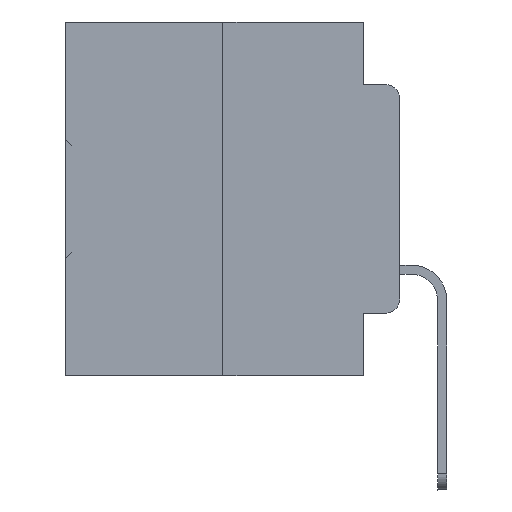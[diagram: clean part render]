
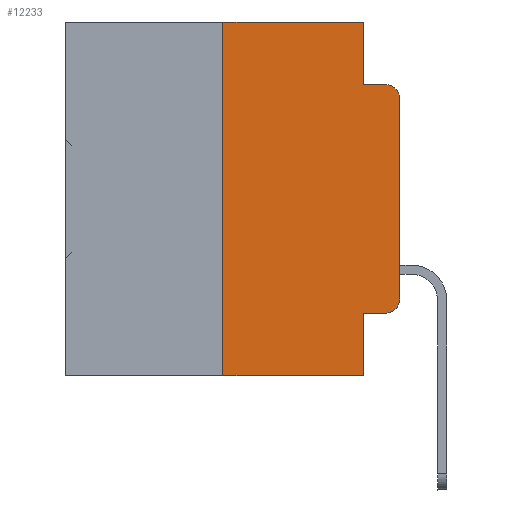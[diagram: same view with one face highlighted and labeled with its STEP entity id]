
A CAD part, left-side view. The second image highlights one B-rep face of the part: STEP entity #12233.
In plain terms, the highlighted planar face has unit normal (-1, 0, 0).
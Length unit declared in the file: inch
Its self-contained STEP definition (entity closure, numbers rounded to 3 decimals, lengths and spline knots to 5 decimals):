
#321 = EDGE_CURVE ( 'NONE', #11624, #19529, #2840, .T. ) ;
#1465 = EDGE_CURVE ( 'NONE', #12386, #24815, #33762, .T. ) ;
#1504 = LINE ( 'NONE', #9749, #30972 ) ;
#1624 = ORIENTED_EDGE ( 'NONE', *, *, #29999, .F. ) ;
#1955 = VERTEX_POINT ( 'NONE', #26578 ) ;
#1976 = ORIENTED_EDGE ( 'NONE', *, *, #26984, .T. ) ;
#2329 = VECTOR ( 'NONE', #22412, 39.37008 ) ;
#2693 = ORIENTED_EDGE ( 'NONE', *, *, #1465, .T. ) ;
#2697 = DIRECTION ( 'NONE',  ( 0., 0., 1. ) ) ;
#2840 = LINE ( 'NONE', #5362, #21229 ) ;
#3437 = EDGE_LOOP ( 'NONE', ( #18092, #22411, #13789, #13077, #34495, #13968, #5350, #1624, #1976, #2693 ) ) ;
#4171 = DIRECTION ( 'NONE',  ( 0., -1., 0. ) ) ;
#4357 = AXIS2_PLACEMENT_3D ( 'NONE', #8572, #22682, #22506 ) ;
#4537 = VECTOR ( 'NONE', #34761, 39.37008 ) ;
#5217 = VECTOR ( 'NONE', #26780, 39.37008 ) ;
#5269 = DIRECTION ( 'NONE',  ( 0., -1., 0. ) ) ;
#5350 = ORIENTED_EDGE ( 'NONE', *, *, #20491, .T. ) ;
#5362 = CARTESIAN_POINT ( 'NONE',  ( 0., 0.473, 0. ) ) ;
#5395 = CARTESIAN_POINT ( 'NONE',  ( 0., 0.25, 0. ) ) ;
#6308 = CARTESIAN_POINT ( 'NONE',  ( 0., 0.051, 0. ) ) ;
#6674 = CARTESIAN_POINT ( 'NONE',  ( 0., 0.051, -0.0885 ) ) ;
#8049 = AXIS2_PLACEMENT_3D ( 'NONE', #9454, #20366, #17683 ) ;
#8396 = DIRECTION ( 'NONE',  ( 0., 0., -1. ) ) ;
#8426 = EDGE_CURVE ( 'NONE', #19529, #9426, #27746, .T. ) ;
#8572 = CARTESIAN_POINT ( 'NONE',  ( 0., 0.02, -0.1085 ) ) ;
#9426 = VERTEX_POINT ( 'NONE', #30774 ) ;
#9454 = CARTESIAN_POINT ( 'NONE',  ( 0., 0.02, -0.3915 ) ) ;
#9749 = CARTESIAN_POINT ( 'NONE',  ( 0., 0.473, -0.5 ) ) ;
#9916 = CARTESIAN_POINT ( 'NONE',  ( 0., 0.051, 0. ) ) ;
#10252 = EDGE_CURVE ( 'NONE', #9426, #20749, #14718, .T. ) ;
#10330 = CARTESIAN_POINT ( 'NONE',  ( 0., 0.051, -0.4115 ) ) ;
#10726 = PLANE ( 'NONE',  #22239 ) ;
#11624 = VERTEX_POINT ( 'NONE', #28161 ) ;
#11834 = VECTOR ( 'NONE', #4171, 39.37008 ) ;
#12233 = ADVANCED_FACE ( 'NONE', ( #16439 ), #10726, .F. ) ;
#12386 = VERTEX_POINT ( 'NONE', #33266 ) ;
#13077 = ORIENTED_EDGE ( 'NONE', *, *, #8426, .F. ) ;
#13789 = ORIENTED_EDGE ( 'NONE', *, *, #10252, .F. ) ;
#13914 = VERTEX_POINT ( 'NONE', #22358 ) ;
#13968 = ORIENTED_EDGE ( 'NONE', *, *, #21806, .F. ) ;
#14221 = VECTOR ( 'NONE', #2697, 39.37008 ) ;
#14718 = LINE ( 'NONE', #6674, #11834 ) ;
#15417 = VERTEX_POINT ( 'NONE', #22706 ) ;
#16270 = DIRECTION ( 'NONE',  ( 0., -1., 0. ) ) ;
#16439 = FACE_OUTER_BOUND ( 'NONE', #3437, .T. ) ;
#17683 = DIRECTION ( 'NONE',  ( 0., 0., -1. ) ) ;
#18092 = ORIENTED_EDGE ( 'NONE', *, *, #19408, .T. ) ;
#18486 = LINE ( 'NONE', #9916, #4537 ) ;
#19408 = EDGE_CURVE ( 'NONE', #24815, #30811, #19719, .T. ) ;
#19529 = VERTEX_POINT ( 'NONE', #6308 ) ;
#19719 = LINE ( 'NONE', #20094, #2329 ) ;
#20094 = CARTESIAN_POINT ( 'NONE',  ( 0., 0., 0. ) ) ;
#20366 = DIRECTION ( 'NONE',  ( -1., 0., 0. ) ) ;
#20491 = EDGE_CURVE ( 'NONE', #13914, #15417, #1504, .T. ) ;
#20749 = VERTEX_POINT ( 'NONE', #30478 ) ;
#21229 = VECTOR ( 'NONE', #16270, 39.37008 ) ;
#21687 = CARTESIAN_POINT ( 'NONE',  ( 0., 0., -0.3915 ) ) ;
#21806 = EDGE_CURVE ( 'NONE', #13914, #11624, #27218, .T. ) ;
#22239 = AXIS2_PLACEMENT_3D ( 'NONE', #30047, #27356, #8396 ) ;
#22358 = CARTESIAN_POINT ( 'NONE',  ( 0., 0.25, -0.5 ) ) ;
#22411 = ORIENTED_EDGE ( 'NONE', *, *, #35269, .T. ) ;
#22412 = DIRECTION ( 'NONE',  ( 0., 0., 1. ) ) ;
#22506 = DIRECTION ( 'NONE',  ( 0., 0., -1. ) ) ;
#22682 = DIRECTION ( 'NONE',  ( -1., 0., 0. ) ) ;
#22706 = CARTESIAN_POINT ( 'NONE',  ( 0., 0.051, -0.5 ) ) ;
#23819 = VECTOR ( 'NONE', #25058, 39.37008 ) ;
#24815 = VERTEX_POINT ( 'NONE', #21687 ) ;
#25058 = DIRECTION ( 'NONE',  ( 0., 0., -1. ) ) ;
#26578 = CARTESIAN_POINT ( 'NONE',  ( 0., 0.051, -0.4115 ) ) ;
#26780 = DIRECTION ( 'NONE',  ( 0., -1., 0. ) ) ;
#26984 = EDGE_CURVE ( 'NONE', #1955, #12386, #32496, .T. ) ;
#27218 = LINE ( 'NONE', #5395, #14221 ) ;
#27356 = DIRECTION ( 'NONE',  ( 1., 0., 0. ) ) ;
#27746 = LINE ( 'NONE', #30615, #23819 ) ;
#28161 = CARTESIAN_POINT ( 'NONE',  ( 0., 0.25, 0. ) ) ;
#29999 = EDGE_CURVE ( 'NONE', #1955, #15417, #18486, .T. ) ;
#30047 = CARTESIAN_POINT ( 'NONE',  ( 0., 0.473, 0. ) ) ;
#30478 = CARTESIAN_POINT ( 'NONE',  ( 0., 0.02, -0.0885 ) ) ;
#30615 = CARTESIAN_POINT ( 'NONE',  ( 0., 0.051, 0. ) ) ;
#30774 = CARTESIAN_POINT ( 'NONE',  ( 0., 0.051, -0.0885 ) ) ;
#30811 = VERTEX_POINT ( 'NONE', #34856 ) ;
#30972 = VECTOR ( 'NONE', #5269, 39.37008 ) ;
#32496 = LINE ( 'NONE', #10330, #5217 ) ;
#33266 = CARTESIAN_POINT ( 'NONE',  ( 0., 0.02, -0.4115 ) ) ;
#33762 = CIRCLE ( 'NONE', #8049, 0.02 ) ;
#34495 = ORIENTED_EDGE ( 'NONE', *, *, #321, .F. ) ;
#34761 = DIRECTION ( 'NONE',  ( 0., 0., -1. ) ) ;
#34856 = CARTESIAN_POINT ( 'NONE',  ( 0., 0., -0.1085 ) ) ;
#35222 = CIRCLE ( 'NONE', #4357, 0.02 ) ;
#35269 = EDGE_CURVE ( 'NONE', #30811, #20749, #35222, .T. ) ;
